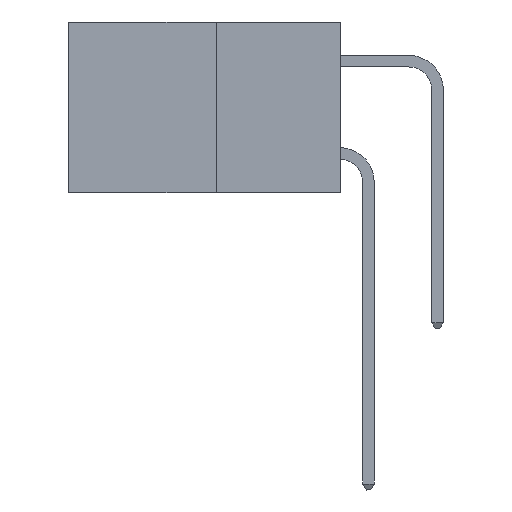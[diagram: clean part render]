
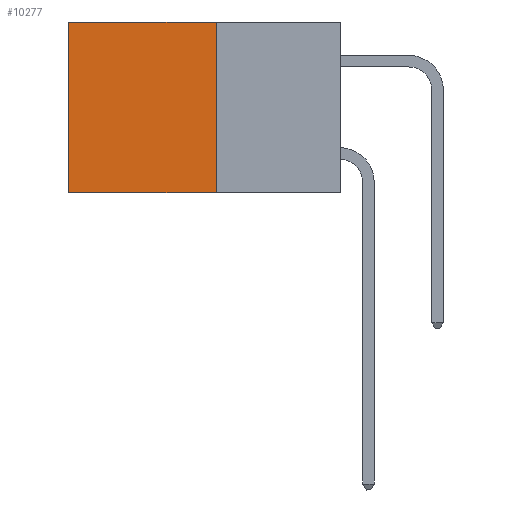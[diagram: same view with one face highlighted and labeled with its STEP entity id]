
A CAD part, left-side view. The second image highlights one B-rep face of the part: STEP entity #10277.
In plain terms, the highlighted planar face has unit normal (-1, 0, 0).
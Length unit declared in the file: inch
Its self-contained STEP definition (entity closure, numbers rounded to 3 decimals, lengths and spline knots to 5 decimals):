
#175 = CARTESIAN_POINT ( 'NONE',  ( 0.277, 0.59, 0. ) ) ;
#269 = DIRECTION ( 'NONE',  ( 0., 1., 0. ) ) ;
#715 = LINE ( 'NONE', #16371, #14654 ) ;
#1797 = CARTESIAN_POINT ( 'NONE',  ( 0.277, 0.27, 0. ) ) ;
#2014 = ORIENTED_EDGE ( 'NONE', *, *, #17686, .F. ) ;
#2276 = ORIENTED_EDGE ( 'NONE', *, *, #15334, .T. ) ;
#3156 = LINE ( 'NONE', #5024, #20196 ) ;
#3374 = DIRECTION ( 'NONE',  ( 0., 0., -1. ) ) ;
#4336 = LINE ( 'NONE', #5391, #17062 ) ;
#4473 = CARTESIAN_POINT ( 'NONE',  ( 0.277, 0.27, -0.37 ) ) ;
#5024 = CARTESIAN_POINT ( 'NONE',  ( 0.277, 0.27, -0.37 ) ) ;
#5391 = CARTESIAN_POINT ( 'NONE',  ( 0.277, 0.27, -0.37 ) ) ;
#5634 = LINE ( 'NONE', #11855, #10618 ) ;
#6190 = DIRECTION ( 'NONE',  ( 0., 0., -1. ) ) ;
#6653 = VERTEX_POINT ( 'NONE', #175 ) ;
#7296 = EDGE_LOOP ( 'NONE', ( #2276, #15972, #2014, #16207 ) ) ;
#8343 = VERTEX_POINT ( 'NONE', #19938 ) ;
#9908 = VERTEX_POINT ( 'NONE', #1797 ) ;
#10277 = ADVANCED_FACE ( 'NONE', ( #16730 ), #12827, .F. ) ;
#10618 = VECTOR ( 'NONE', #3374, 39.37008 ) ;
#11855 = CARTESIAN_POINT ( 'NONE',  ( 0.277, 0.59, -0.37 ) ) ;
#11910 = AXIS2_PLACEMENT_3D ( 'NONE', #4473, #16097, #6190 ) ;
#12827 = PLANE ( 'NONE',  #11910 ) ;
#13425 = DIRECTION ( 'NONE',  ( 0., 0., -1. ) ) ;
#14654 = VECTOR ( 'NONE', #21202, 39.37008 ) ;
#15334 = EDGE_CURVE ( 'NONE', #6653, #8343, #5634, .T. ) ;
#15972 = ORIENTED_EDGE ( 'NONE', *, *, #21144, .F. ) ;
#16097 = DIRECTION ( 'NONE',  ( 1., 0., 0. ) ) ;
#16207 = ORIENTED_EDGE ( 'NONE', *, *, #16896, .T. ) ;
#16371 = CARTESIAN_POINT ( 'NONE',  ( 0.277, 0.27, 0. ) ) ;
#16730 = FACE_OUTER_BOUND ( 'NONE', #7296, .T. ) ;
#16896 = EDGE_CURVE ( 'NONE', #9908, #6653, #715, .T. ) ;
#17062 = VECTOR ( 'NONE', #269, 39.37008 ) ;
#17250 = CARTESIAN_POINT ( 'NONE',  ( 0.277, 0.27, -0.37 ) ) ;
#17686 = EDGE_CURVE ( 'NONE', #9908, #19351, #3156, .T. ) ;
#19351 = VERTEX_POINT ( 'NONE', #17250 ) ;
#19938 = CARTESIAN_POINT ( 'NONE',  ( 0.277, 0.59, -0.37 ) ) ;
#20196 = VECTOR ( 'NONE', #13425, 39.37008 ) ;
#21144 = EDGE_CURVE ( 'NONE', #19351, #8343, #4336, .T. ) ;
#21202 = DIRECTION ( 'NONE',  ( 0., 1., 0. ) ) ;
